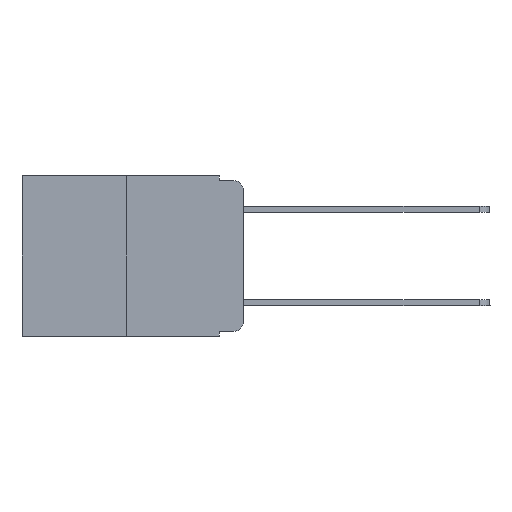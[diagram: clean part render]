
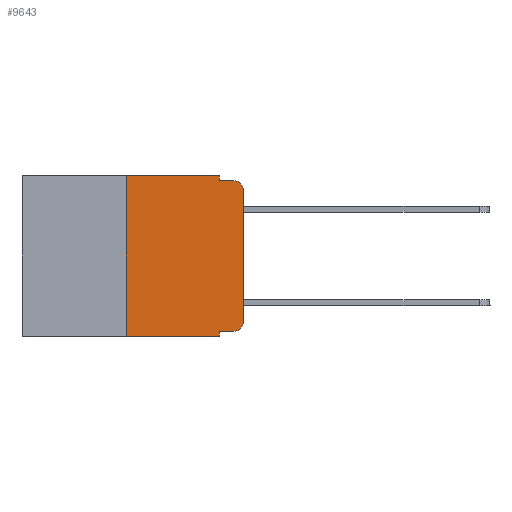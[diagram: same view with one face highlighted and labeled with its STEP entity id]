
A CAD part, left-side view. The second image highlights one B-rep face of the part: STEP entity #9643.
In plain terms, the highlighted planar face has unit normal (-1, 0, 0).
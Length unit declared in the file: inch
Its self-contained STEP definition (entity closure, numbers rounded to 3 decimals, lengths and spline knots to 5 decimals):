
#134 = ORIENTED_EDGE ( 'NONE', *, *, #10179, .T. ) ;
#303 = CARTESIAN_POINT ( 'NONE',  ( 0., 0.473, -0.343 ) ) ;
#797 = DIRECTION ( 'NONE',  ( 0., 0., -1. ) ) ;
#1040 = DIRECTION ( 'NONE',  ( -1., 0., 0. ) ) ;
#1076 = CARTESIAN_POINT ( 'NONE',  ( 0., 0.473, 0. ) ) ;
#1156 = DIRECTION ( 'NONE',  ( 0., 0., -1. ) ) ;
#1668 = LINE ( 'NONE', #15077, #17130 ) ;
#1705 = ORIENTED_EDGE ( 'NONE', *, *, #10287, .T. ) ;
#2154 = VERTEX_POINT ( 'NONE', #13914 ) ;
#2432 = EDGE_CURVE ( 'NONE', #2581, #3816, #1668, .T. ) ;
#2454 = ORIENTED_EDGE ( 'NONE', *, *, #7334, .F. ) ;
#2521 = ORIENTED_EDGE ( 'NONE', *, *, #3801, .F. ) ;
#2581 = VERTEX_POINT ( 'NONE', #10851 ) ;
#3098 = VERTEX_POINT ( 'NONE', #17407 ) ;
#3270 = VERTEX_POINT ( 'NONE', #18472 ) ;
#3475 = VERTEX_POINT ( 'NONE', #13911 ) ;
#3668 = LINE ( 'NONE', #13226, #18260 ) ;
#3801 = EDGE_CURVE ( 'NONE', #11589, #8435, #12253, .T. ) ;
#3808 = EDGE_LOOP ( 'NONE', ( #14354, #6859, #2521, #17739, #19060, #15510, #13361, #2454, #1705, #134 ) ) ;
#3816 = VERTEX_POINT ( 'NONE', #10017 ) ;
#3853 = DIRECTION ( 'NONE',  ( 0., 0., -1. ) ) ;
#3904 = DIRECTION ( 'NONE',  ( 0., 0., 1. ) ) ;
#4138 = DIRECTION ( 'NONE',  ( 0., 0., -1. ) ) ;
#4252 = CARTESIAN_POINT ( 'NONE',  ( 0., 0.02, -0.313 ) ) ;
#4342 = CARTESIAN_POINT ( 'NONE',  ( 0., 0.25, 0. ) ) ;
#4382 = PLANE ( 'NONE',  #4823 ) ;
#4507 = VECTOR ( 'NONE', #18126, 39.37008 ) ;
#4780 = DIRECTION ( 'NONE',  ( 0., -1., 0. ) ) ;
#4823 = AXIS2_PLACEMENT_3D ( 'NONE', #1076, #20959, #15766 ) ;
#4833 = AXIS2_PLACEMENT_3D ( 'NONE', #4252, #10895, #1156 ) ;
#4835 = CIRCLE ( 'NONE', #9289, 0.02 ) ;
#4886 = LINE ( 'NONE', #303, #6993 ) ;
#5137 = LINE ( 'NONE', #15121, #5160 ) ;
#5160 = VECTOR ( 'NONE', #18499, 39.37008 ) ;
#5588 = VECTOR ( 'NONE', #9066, 39.37008 ) ;
#6859 = ORIENTED_EDGE ( 'NONE', *, *, #8196, .T. ) ;
#6993 = VECTOR ( 'NONE', #4780, 39.37008 ) ;
#7183 = VECTOR ( 'NONE', #797, 39.37008 ) ;
#7334 = EDGE_CURVE ( 'NONE', #13124, #3475, #17451, .T. ) ;
#7598 = LINE ( 'NONE', #20225, #9345 ) ;
#7750 = CARTESIAN_POINT ( 'NONE',  ( 0., 0.25, -0.343 ) ) ;
#8196 = EDGE_CURVE ( 'NONE', #3816, #8435, #4835, .T. ) ;
#8435 = VERTEX_POINT ( 'NONE', #16913 ) ;
#9066 = DIRECTION ( 'NONE',  ( 0., 0., 1. ) ) ;
#9289 = AXIS2_PLACEMENT_3D ( 'NONE', #19003, #1040, #4138 ) ;
#9345 = VECTOR ( 'NONE', #3853, 39.37008 ) ;
#9401 = EDGE_CURVE ( 'NONE', #2154, #3098, #5137, .T. ) ;
#9643 = ADVANCED_FACE ( 'NONE', ( #10822 ), #4382, .F. ) ;
#10017 = CARTESIAN_POINT ( 'NONE',  ( 0., 0., -0.03 ) ) ;
#10179 = EDGE_CURVE ( 'NONE', #3270, #2581, #10677, .T. ) ;
#10287 = EDGE_CURVE ( 'NONE', #13124, #3270, #3668, .T. ) ;
#10670 = LINE ( 'NONE', #4342, #5588 ) ;
#10677 = CIRCLE ( 'NONE', #4833, 0.02 ) ;
#10822 = FACE_OUTER_BOUND ( 'NONE', #3808, .T. ) ;
#10851 = CARTESIAN_POINT ( 'NONE',  ( 0., 0., -0.313 ) ) ;
#10895 = DIRECTION ( 'NONE',  ( -1., 0., 0. ) ) ;
#11589 = VERTEX_POINT ( 'NONE', #12479 ) ;
#12152 = CARTESIAN_POINT ( 'NONE',  ( 0., 0.051, 0. ) ) ;
#12253 = LINE ( 'NONE', #13245, #4507 ) ;
#12333 = EDGE_CURVE ( 'NONE', #16179, #2154, #10670, .T. ) ;
#12479 = CARTESIAN_POINT ( 'NONE',  ( 0., 0.051, -0.01 ) ) ;
#13124 = VERTEX_POINT ( 'NONE', #18408 ) ;
#13226 = CARTESIAN_POINT ( 'NONE',  ( 0., 0.051, -0.333 ) ) ;
#13245 = CARTESIAN_POINT ( 'NONE',  ( 0., 0.051, -0.01 ) ) ;
#13361 = ORIENTED_EDGE ( 'NONE', *, *, #20780, .T. ) ;
#13911 = CARTESIAN_POINT ( 'NONE',  ( 0., 0.051, -0.343 ) ) ;
#13914 = CARTESIAN_POINT ( 'NONE',  ( 0., 0.25, 0. ) ) ;
#14354 = ORIENTED_EDGE ( 'NONE', *, *, #2432, .T. ) ;
#15077 = CARTESIAN_POINT ( 'NONE',  ( 0., 0., 0. ) ) ;
#15121 = CARTESIAN_POINT ( 'NONE',  ( 0., 0.473, 0. ) ) ;
#15510 = ORIENTED_EDGE ( 'NONE', *, *, #12333, .F. ) ;
#15766 = DIRECTION ( 'NONE',  ( 0., 0., -1. ) ) ;
#16179 = VERTEX_POINT ( 'NONE', #7750 ) ;
#16913 = CARTESIAN_POINT ( 'NONE',  ( 0., 0.02, -0.01 ) ) ;
#17130 = VECTOR ( 'NONE', #3904, 39.37008 ) ;
#17407 = CARTESIAN_POINT ( 'NONE',  ( 0., 0.051, 0. ) ) ;
#17451 = LINE ( 'NONE', #12152, #7183 ) ;
#17739 = ORIENTED_EDGE ( 'NONE', *, *, #18359, .F. ) ;
#18126 = DIRECTION ( 'NONE',  ( 0., -1., 0. ) ) ;
#18260 = VECTOR ( 'NONE', #19831, 39.37008 ) ;
#18359 = EDGE_CURVE ( 'NONE', #3098, #11589, #7598, .T. ) ;
#18408 = CARTESIAN_POINT ( 'NONE',  ( 0., 0.051, -0.333 ) ) ;
#18472 = CARTESIAN_POINT ( 'NONE',  ( 0., 0.02, -0.333 ) ) ;
#18499 = DIRECTION ( 'NONE',  ( 0., -1., 0. ) ) ;
#19003 = CARTESIAN_POINT ( 'NONE',  ( 0., 0.02, -0.03 ) ) ;
#19060 = ORIENTED_EDGE ( 'NONE', *, *, #9401, .F. ) ;
#19831 = DIRECTION ( 'NONE',  ( 0., -1., 0. ) ) ;
#20225 = CARTESIAN_POINT ( 'NONE',  ( 0., 0.051, 0. ) ) ;
#20780 = EDGE_CURVE ( 'NONE', #16179, #3475, #4886, .T. ) ;
#20959 = DIRECTION ( 'NONE',  ( 1., 0., 0. ) ) ;
